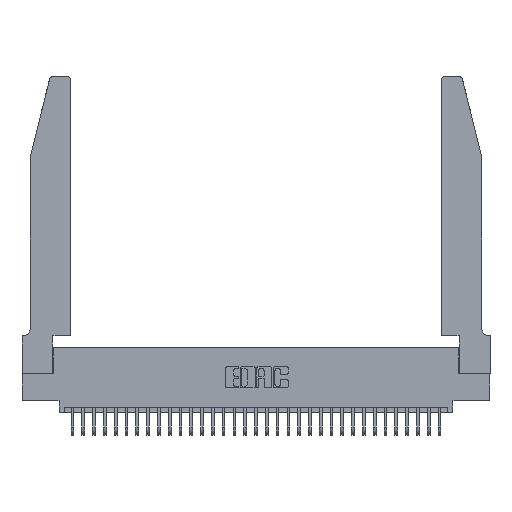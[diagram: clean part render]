
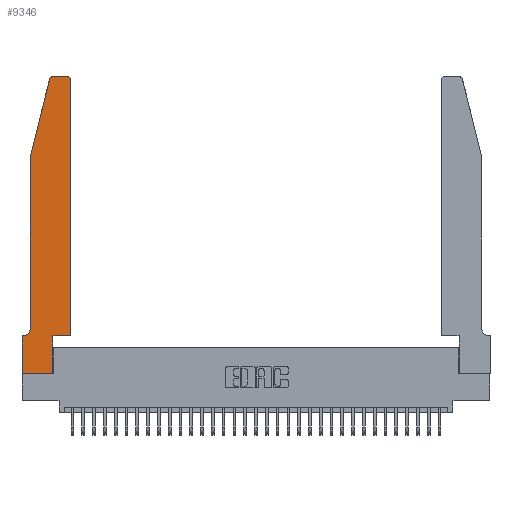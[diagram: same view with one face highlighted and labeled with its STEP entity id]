
A CAD part, top view. The second image highlights one B-rep face of the part: STEP entity #9346.
In plain terms, the highlighted planar face has unit normal (0, 0, 1).
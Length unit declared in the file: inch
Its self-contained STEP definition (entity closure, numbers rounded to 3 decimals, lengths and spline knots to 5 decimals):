
#60 = CARTESIAN_POINT ( 'NONE',  ( 0.4205, 2.72, 0.37 ) ) ;
#175 = CIRCLE ( 'NONE', #21435, 0.03 ) ;
#275 = AXIS2_PLACEMENT_3D ( 'NONE', #22017, #22256, #19023 ) ;
#410 = DIRECTION ( 'NONE',  ( 0., 1., 0. ) ) ;
#1114 = CARTESIAN_POINT ( 'NONE',  ( 0.284, 2.72, 0.37 ) ) ;
#1464 = EDGE_CURVE ( 'NONE', #12031, #14569, #24106, .T. ) ;
#1597 = VECTOR ( 'NONE', #29296, 39.37008 ) ;
#3789 = CARTESIAN_POINT ( 'NONE',  ( 0.25487, 2.72718, 0.37 ) ) ;
#4457 = EDGE_CURVE ( 'NONE', #31648, #14315, #17064, .T. ) ;
#4581 = CARTESIAN_POINT ( 'NONE',  ( 0.0755, 0.35, 0.37 ) ) ;
#4663 = LINE ( 'NONE', #31432, #33782 ) ;
#4807 = EDGE_CURVE ( 'NONE', #14569, #31648, #12409, .T. ) ;
#5526 = EDGE_CURVE ( 'NONE', #14315, #34427, #11933, .T. ) ;
#6464 = DIRECTION ( 'NONE',  ( 1., 0., 0. ) ) ;
#6586 = DIRECTION ( 'NONE',  ( 0., 0., 1. ) ) ;
#6887 = ORIENTED_EDGE ( 'NONE', *, *, #7179, .T. ) ;
#7179 = EDGE_CURVE ( 'NONE', #14872, #13345, #11387, .T. ) ;
#7503 = CARTESIAN_POINT ( 'NONE',  ( 0.0755, 0.42, 0.37 ) ) ;
#8213 = CARTESIAN_POINT ( 'NONE',  ( 0., 0., 0.37 ) ) ;
#8497 = CARTESIAN_POINT ( 'NONE',  ( 0., 0., 0.37 ) ) ;
#9346 = ADVANCED_FACE ( 'NONE', ( #17635 ), #21467, .T. ) ;
#9559 = CARTESIAN_POINT ( 'NONE',  ( 0.2865, 0.35, 0.37 ) ) ;
#9680 = CARTESIAN_POINT ( 'NONE',  ( 0.0055, 0.42, 0.37 ) ) ;
#10078 = DIRECTION ( 'NONE',  ( -1., 0., 0. ) ) ;
#10473 = CARTESIAN_POINT ( 'NONE',  ( 0.0755, 2., 0.37 ) ) ;
#10595 = CARTESIAN_POINT ( 'NONE',  ( 0.0055, 0.35, 0.37 ) ) ;
#11035 = EDGE_CURVE ( 'NONE', #33567, #25364, #4663, .T. ) ;
#11061 = VECTOR ( 'NONE', #32621, 39.37008 ) ;
#11387 = LINE ( 'NONE', #10473, #1597 ) ;
#11933 = LINE ( 'NONE', #19669, #27890 ) ;
#11962 = VECTOR ( 'NONE', #16693, 39.37008 ) ;
#11994 = VERTEX_POINT ( 'NONE', #3789 ) ;
#12031 = VERTEX_POINT ( 'NONE', #14755 ) ;
#12132 = CARTESIAN_POINT ( 'NONE',  ( 0.4505, 2.72, 0.37 ) ) ;
#12153 = ORIENTED_EDGE ( 'NONE', *, *, #4807, .T. ) ;
#12409 = LINE ( 'NONE', #8497, #13236 ) ;
#12410 = DIRECTION ( 'NONE',  ( -1., 0., 0. ) ) ;
#13142 = DIRECTION ( 'NONE',  ( 1., 0., 0. ) ) ;
#13236 = VECTOR ( 'NONE', #27126, 39.37008 ) ;
#13345 = VERTEX_POINT ( 'NONE', #7503 ) ;
#13482 = CIRCLE ( 'NONE', #23480, 0.03 ) ;
#13748 = CARTESIAN_POINT ( 'NONE',  ( 0.0755, 2., 0.37 ) ) ;
#13761 = EDGE_CURVE ( 'NONE', #34427, #14064, #18488, .T. ) ;
#13837 = ORIENTED_EDGE ( 'NONE', *, *, #4457, .T. ) ;
#14064 = VERTEX_POINT ( 'NONE', #12132 ) ;
#14238 = EDGE_CURVE ( 'NONE', #19237, #12031, #19269, .T. ) ;
#14315 = VERTEX_POINT ( 'NONE', #21032 ) ;
#14569 = VERTEX_POINT ( 'NONE', #23204 ) ;
#14755 = CARTESIAN_POINT ( 'NONE',  ( 0., 0.35, 0.37 ) ) ;
#14872 = VERTEX_POINT ( 'NONE', #28840 ) ;
#16073 = ORIENTED_EDGE ( 'NONE', *, *, #24552, .T. ) ;
#16236 = EDGE_CURVE ( 'NONE', #25364, #11994, #13482, .T. ) ;
#16693 = DIRECTION ( 'NONE',  ( -0.239, -0.971, 0. ) ) ;
#17064 = LINE ( 'NONE', #9559, #22068 ) ;
#17257 = ORIENTED_EDGE ( 'NONE', *, *, #14238, .T. ) ;
#17635 = FACE_OUTER_BOUND ( 'NONE', #18719, .T. ) ;
#17737 = DIRECTION ( 'NONE',  ( 0., 0., 1. ) ) ;
#18415 = VECTOR ( 'NONE', #10078, 39.37008 ) ;
#18488 = LINE ( 'NONE', #30309, #31525 ) ;
#18719 = EDGE_LOOP ( 'NONE', ( #25977, #25934, #34932, #6887, #16073, #17257, #33213, #12153, #13837, #23084, #32894, #19976 ) ) ;
#19023 = DIRECTION ( 'NONE',  ( 1., 0., 0. ) ) ;
#19190 = CARTESIAN_POINT ( 'NONE',  ( 0.2865, 0., 0.37 ) ) ;
#19237 = VERTEX_POINT ( 'NONE', #10595 ) ;
#19269 = LINE ( 'NONE', #4581, #18415 ) ;
#19669 = CARTESIAN_POINT ( 'NONE',  ( 0.4505, 0.35, 0.37 ) ) ;
#19976 = ORIENTED_EDGE ( 'NONE', *, *, #26008, .T. ) ;
#20055 = AXIS2_PLACEMENT_3D ( 'NONE', #9680, #28507, #12410 ) ;
#20355 = DIRECTION ( 'NONE',  ( -1., 0., 0. ) ) ;
#21032 = CARTESIAN_POINT ( 'NONE',  ( 0.2865, 0.35, 0.37 ) ) ;
#21435 = AXIS2_PLACEMENT_3D ( 'NONE', #60, #17737, #13142 ) ;
#21467 = PLANE ( 'NONE',  #275 ) ;
#22017 = CARTESIAN_POINT ( 'NONE',  ( 0., 0.35, 0.37 ) ) ;
#22068 = VECTOR ( 'NONE', #25666, 39.37008 ) ;
#22256 = DIRECTION ( 'NONE',  ( 0., 0., 1. ) ) ;
#23084 = ORIENTED_EDGE ( 'NONE', *, *, #5526, .T. ) ;
#23204 = CARTESIAN_POINT ( 'NONE',  ( 0., 0., 0.37 ) ) ;
#23480 = AXIS2_PLACEMENT_3D ( 'NONE', #1114, #6586, #6464 ) ;
#23830 = CARTESIAN_POINT ( 'NONE',  ( 0.4505, 0.35, 0.37 ) ) ;
#23846 = CARTESIAN_POINT ( 'NONE',  ( 0.284, 2.75, 0.37 ) ) ;
#24106 = LINE ( 'NONE', #8213, #11061 ) ;
#24552 = EDGE_CURVE ( 'NONE', #13345, #19237, #34869, .T. ) ;
#25364 = VERTEX_POINT ( 'NONE', #23846 ) ;
#25666 = DIRECTION ( 'NONE',  ( 0., 1., 0. ) ) ;
#25934 = ORIENTED_EDGE ( 'NONE', *, *, #16236, .T. ) ;
#25977 = ORIENTED_EDGE ( 'NONE', *, *, #11035, .T. ) ;
#26008 = EDGE_CURVE ( 'NONE', #14064, #33567, #175, .T. ) ;
#27126 = DIRECTION ( 'NONE',  ( 1., 0., 0. ) ) ;
#27890 = VECTOR ( 'NONE', #33280, 39.37008 ) ;
#28507 = DIRECTION ( 'NONE',  ( 0., 0., -1. ) ) ;
#28728 = CARTESIAN_POINT ( 'NONE',  ( 0.4205, 2.75, 0.37 ) ) ;
#28840 = CARTESIAN_POINT ( 'NONE',  ( 0.0755, 2., 0.37 ) ) ;
#29296 = DIRECTION ( 'NONE',  ( 0., -1., 0. ) ) ;
#30309 = CARTESIAN_POINT ( 'NONE',  ( 0.4505, 0.35, 0.37 ) ) ;
#31432 = CARTESIAN_POINT ( 'NONE',  ( 0.2605, 2.75, 0.37 ) ) ;
#31525 = VECTOR ( 'NONE', #410, 39.37008 ) ;
#31648 = VERTEX_POINT ( 'NONE', #19190 ) ;
#32621 = DIRECTION ( 'NONE',  ( 0., -1., 0. ) ) ;
#32629 = EDGE_CURVE ( 'NONE', #11994, #14872, #33397, .T. ) ;
#32894 = ORIENTED_EDGE ( 'NONE', *, *, #13761, .T. ) ;
#33213 = ORIENTED_EDGE ( 'NONE', *, *, #1464, .T. ) ;
#33280 = DIRECTION ( 'NONE',  ( 1., 0., 0. ) ) ;
#33397 = LINE ( 'NONE', #13748, #11962 ) ;
#33567 = VERTEX_POINT ( 'NONE', #28728 ) ;
#33782 = VECTOR ( 'NONE', #20355, 39.37008 ) ;
#34427 = VERTEX_POINT ( 'NONE', #23830 ) ;
#34869 = CIRCLE ( 'NONE', #20055, 0.07 ) ;
#34932 = ORIENTED_EDGE ( 'NONE', *, *, #32629, .T. ) ;
